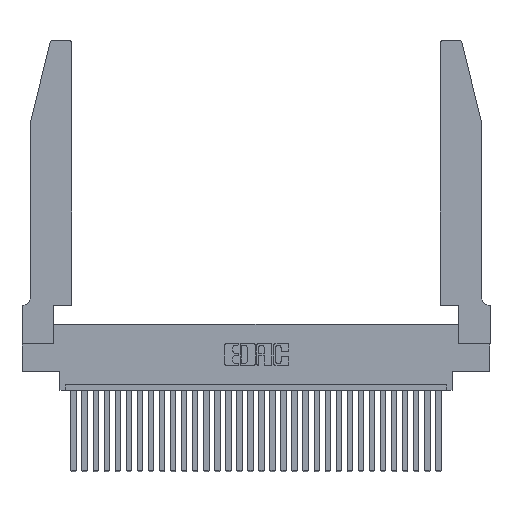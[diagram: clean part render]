
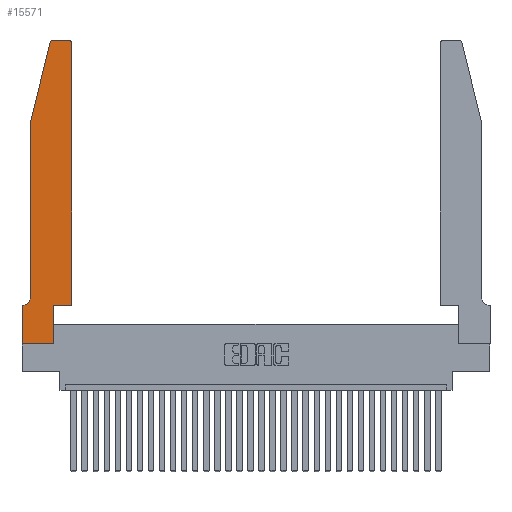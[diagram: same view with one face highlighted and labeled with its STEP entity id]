
A CAD part, top view. The second image highlights one B-rep face of the part: STEP entity #15571.
In plain terms, the highlighted planar face has unit normal (0, 0, 1).
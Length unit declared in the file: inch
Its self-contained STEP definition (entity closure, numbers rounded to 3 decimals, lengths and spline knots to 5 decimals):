
#84 = ORIENTED_EDGE ( 'NONE', *, *, #13701, .T. ) ;
#121 = ORIENTED_EDGE ( 'NONE', *, *, #24122, .T. ) ;
#160 = VECTOR ( 'NONE', #24672, 39.37008 ) ;
#525 = DIRECTION ( 'NONE',  ( 0., 1., 0. ) ) ;
#1490 = CARTESIAN_POINT ( 'NONE',  ( 0.284, 2.72, 0.37 ) ) ;
#1513 = LINE ( 'NONE', #5766, #22391 ) ;
#1916 = DIRECTION ( 'NONE',  ( 1., 0., 0. ) ) ;
#2049 = VERTEX_POINT ( 'NONE', #19644 ) ;
#2276 = ORIENTED_EDGE ( 'NONE', *, *, #11397, .T. ) ;
#2443 = CARTESIAN_POINT ( 'NONE',  ( 0.0055, 0.42, 0.37 ) ) ;
#3094 = CARTESIAN_POINT ( 'NONE',  ( 0.25487, 2.72718, 0.37 ) ) ;
#3187 = LINE ( 'NONE', #24811, #16131 ) ;
#3957 = EDGE_CURVE ( 'NONE', #7275, #25680, #16576, .T. ) ;
#5072 = CARTESIAN_POINT ( 'NONE',  ( 0.4505, 0.35, 0.37 ) ) ;
#5130 = VECTOR ( 'NONE', #29355, 39.37008 ) ;
#5232 = CARTESIAN_POINT ( 'NONE',  ( 0.4505, 0.35, 0.37 ) ) ;
#5279 = EDGE_CURVE ( 'NONE', #25201, #2049, #25346, .T. ) ;
#5460 = DIRECTION ( 'NONE',  ( 1., 0., 0. ) ) ;
#5766 = CARTESIAN_POINT ( 'NONE',  ( 0., 0., 0.37 ) ) ;
#5829 = AXIS2_PLACEMENT_3D ( 'NONE', #2443, #15042, #14938 ) ;
#6266 = ORIENTED_EDGE ( 'NONE', *, *, #11309, .T. ) ;
#7031 = CARTESIAN_POINT ( 'NONE',  ( 0.4205, 2.75, 0.37 ) ) ;
#7120 = CIRCLE ( 'NONE', #12647, 0.03 ) ;
#7275 = VERTEX_POINT ( 'NONE', #16699 ) ;
#7426 = VERTEX_POINT ( 'NONE', #25722 ) ;
#7926 = VERTEX_POINT ( 'NONE', #28112 ) ;
#8213 = ORIENTED_EDGE ( 'NONE', *, *, #15435, .T. ) ;
#8564 = EDGE_CURVE ( 'NONE', #8696, #7275, #1513, .T. ) ;
#8696 = VERTEX_POINT ( 'NONE', #21557 ) ;
#9017 = DIRECTION ( 'NONE',  ( 0., 0., 1. ) ) ;
#9255 = LINE ( 'NONE', #5232, #25981 ) ;
#9376 = VERTEX_POINT ( 'NONE', #25409 ) ;
#9390 = VERTEX_POINT ( 'NONE', #22533 ) ;
#10100 = CARTESIAN_POINT ( 'NONE',  ( 0.0755, 2., 0.37 ) ) ;
#10147 = FACE_OUTER_BOUND ( 'NONE', #23060, .T. ) ;
#10866 = DIRECTION ( 'NONE',  ( 0., -1., 0. ) ) ;
#11309 = EDGE_CURVE ( 'NONE', #25680, #23116, #28654, .T. ) ;
#11325 = ORIENTED_EDGE ( 'NONE', *, *, #12908, .T. ) ;
#11397 = EDGE_CURVE ( 'NONE', #20676, #9376, #3187, .T. ) ;
#11423 = AXIS2_PLACEMENT_3D ( 'NONE', #1490, #9017, #1916 ) ;
#11982 = ORIENTED_EDGE ( 'NONE', *, *, #24754, .T. ) ;
#12647 = AXIS2_PLACEMENT_3D ( 'NONE', #18989, #22039, #15437 ) ;
#12908 = EDGE_CURVE ( 'NONE', #2049, #18768, #22487, .T. ) ;
#12914 = CARTESIAN_POINT ( 'NONE',  ( 0.0755, 0.35, 0.37 ) ) ;
#12931 = DIRECTION ( 'NONE',  ( 0., -1., 0. ) ) ;
#13048 = DIRECTION ( 'NONE',  ( 1., 0., 0. ) ) ;
#13701 = EDGE_CURVE ( 'NONE', #7926, #8696, #19770, .T. ) ;
#14938 = DIRECTION ( 'NONE',  ( -1., 0., 0. ) ) ;
#15042 = DIRECTION ( 'NONE',  ( 0., 0., -1. ) ) ;
#15320 = DIRECTION ( 'NONE',  ( 1., 0., 0. ) ) ;
#15435 = EDGE_CURVE ( 'NONE', #9376, #25201, #7120, .T. ) ;
#15437 = DIRECTION ( 'NONE',  ( 1., 0., 0. ) ) ;
#15571 = ADVANCED_FACE ( 'NONE', ( #10147 ), #17859, .T. ) ;
#16131 = VECTOR ( 'NONE', #525, 39.37008 ) ;
#16568 = EDGE_CURVE ( 'NONE', #9390, #7426, #26810, .T. ) ;
#16576 = LINE ( 'NONE', #22317, #25712 ) ;
#16699 = CARTESIAN_POINT ( 'NONE',  ( 0., 0., 0.37 ) ) ;
#17217 = LINE ( 'NONE', #10100, #160 ) ;
#17356 = DIRECTION ( 'NONE',  ( -1., 0., 0. ) ) ;
#17696 = ORIENTED_EDGE ( 'NONE', *, *, #16568, .T. ) ;
#17859 = PLANE ( 'NONE',  #18577 ) ;
#18003 = CARTESIAN_POINT ( 'NONE',  ( 0.2865, 0.35, 0.37 ) ) ;
#18264 = VECTOR ( 'NONE', #17356, 39.37008 ) ;
#18577 = AXIS2_PLACEMENT_3D ( 'NONE', #30208, #25180, #13048 ) ;
#18768 = VERTEX_POINT ( 'NONE', #3094 ) ;
#18989 = CARTESIAN_POINT ( 'NONE',  ( 0.4205, 2.72, 0.37 ) ) ;
#19294 = CARTESIAN_POINT ( 'NONE',  ( 0.2865, 0., 0.37 ) ) ;
#19644 = CARTESIAN_POINT ( 'NONE',  ( 0.284, 2.75, 0.37 ) ) ;
#19770 = LINE ( 'NONE', #12914, #18264 ) ;
#20368 = VECTOR ( 'NONE', #12931, 39.37008 ) ;
#20676 = VERTEX_POINT ( 'NONE', #5072 ) ;
#21557 = CARTESIAN_POINT ( 'NONE',  ( 0., 0.35, 0.37 ) ) ;
#21856 = EDGE_CURVE ( 'NONE', #18768, #9390, #17217, .T. ) ;
#22026 = ORIENTED_EDGE ( 'NONE', *, *, #8564, .T. ) ;
#22039 = DIRECTION ( 'NONE',  ( 0., 0., 1. ) ) ;
#22317 = CARTESIAN_POINT ( 'NONE',  ( 0., 0., 0.37 ) ) ;
#22391 = VECTOR ( 'NONE', #10866, 39.37008 ) ;
#22487 = CIRCLE ( 'NONE', #11423, 0.03 ) ;
#22533 = CARTESIAN_POINT ( 'NONE',  ( 0.0755, 2., 0.37 ) ) ;
#23060 = EDGE_LOOP ( 'NONE', ( #25217, #11325, #24795, #17696, #121, #84, #22026, #27565, #6266, #11982, #2276, #8213 ) ) ;
#23116 = VERTEX_POINT ( 'NONE', #27446 ) ;
#24122 = EDGE_CURVE ( 'NONE', #7426, #7926, #29174, .T. ) ;
#24126 = VECTOR ( 'NONE', #29836, 39.37008 ) ;
#24672 = DIRECTION ( 'NONE',  ( -0.239, -0.971, 0. ) ) ;
#24754 = EDGE_CURVE ( 'NONE', #23116, #20676, #9255, .T. ) ;
#24795 = ORIENTED_EDGE ( 'NONE', *, *, #21856, .T. ) ;
#24811 = CARTESIAN_POINT ( 'NONE',  ( 0.4505, 0.35, 0.37 ) ) ;
#25180 = DIRECTION ( 'NONE',  ( 0., 0., 1. ) ) ;
#25201 = VERTEX_POINT ( 'NONE', #7031 ) ;
#25217 = ORIENTED_EDGE ( 'NONE', *, *, #5279, .T. ) ;
#25346 = LINE ( 'NONE', #29257, #5130 ) ;
#25409 = CARTESIAN_POINT ( 'NONE',  ( 0.4505, 2.72, 0.37 ) ) ;
#25680 = VERTEX_POINT ( 'NONE', #19294 ) ;
#25712 = VECTOR ( 'NONE', #15320, 39.37008 ) ;
#25722 = CARTESIAN_POINT ( 'NONE',  ( 0.0755, 0.42, 0.37 ) ) ;
#25981 = VECTOR ( 'NONE', #5460, 39.37008 ) ;
#26810 = LINE ( 'NONE', #29559, #20368 ) ;
#27446 = CARTESIAN_POINT ( 'NONE',  ( 0.2865, 0.35, 0.37 ) ) ;
#27565 = ORIENTED_EDGE ( 'NONE', *, *, #3957, .T. ) ;
#28112 = CARTESIAN_POINT ( 'NONE',  ( 0.0055, 0.35, 0.37 ) ) ;
#28654 = LINE ( 'NONE', #18003, #24126 ) ;
#29174 = CIRCLE ( 'NONE', #5829, 0.07 ) ;
#29257 = CARTESIAN_POINT ( 'NONE',  ( 0.2605, 2.75, 0.37 ) ) ;
#29355 = DIRECTION ( 'NONE',  ( -1., 0., 0. ) ) ;
#29559 = CARTESIAN_POINT ( 'NONE',  ( 0.0755, 2., 0.37 ) ) ;
#29836 = DIRECTION ( 'NONE',  ( 0., 1., 0. ) ) ;
#30208 = CARTESIAN_POINT ( 'NONE',  ( 0., 0.35, 0.37 ) ) ;
